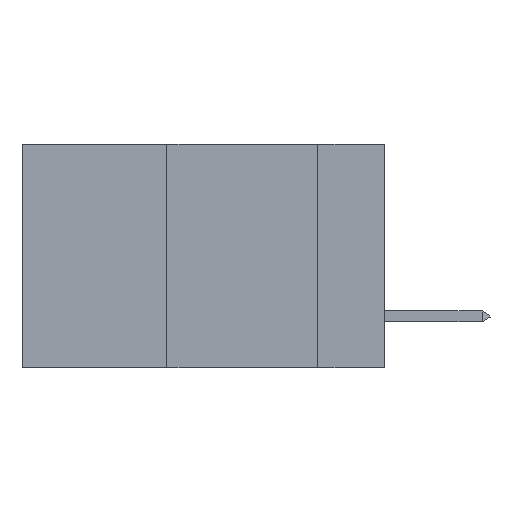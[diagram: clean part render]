
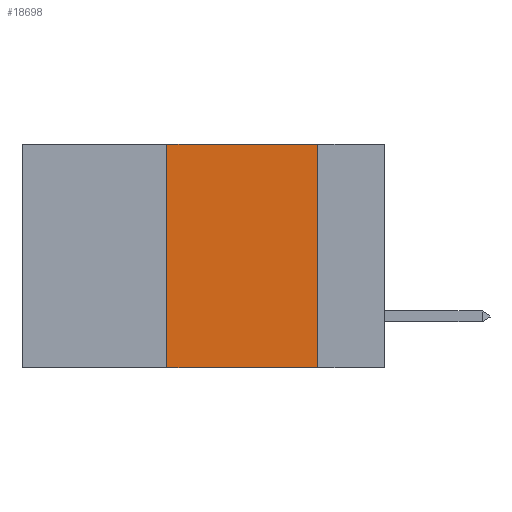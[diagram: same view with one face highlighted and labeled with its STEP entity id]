
A CAD part, left-side view. The second image highlights one B-rep face of the part: STEP entity #18698.
In plain terms, the highlighted planar face has unit normal (-1, 0, 0).
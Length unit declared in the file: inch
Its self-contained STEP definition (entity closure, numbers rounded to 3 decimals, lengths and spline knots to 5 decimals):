
#898 = EDGE_LOOP ( 'NONE', ( #26994, #12466, #18813, #14723 ) ) ;
#1641 = VECTOR ( 'NONE', #14928, 39.37008 ) ;
#2101 = DIRECTION ( 'NONE',  ( 0., -1., 0. ) ) ;
#3492 = CARTESIAN_POINT ( 'NONE',  ( 0., 0.36, 0. ) ) ;
#4423 = PLANE ( 'NONE',  #25157 ) ;
#5091 = VERTEX_POINT ( 'NONE', #13946 ) ;
#5273 = EDGE_CURVE ( 'NONE', #17219, #12558, #10427, .T. ) ;
#7142 = DIRECTION ( 'NONE',  ( 0., 0., -1. ) ) ;
#8526 = VECTOR ( 'NONE', #16353, 39.37008 ) ;
#9247 = CARTESIAN_POINT ( 'NONE',  ( 0., 0.11, -0.37 ) ) ;
#10427 = LINE ( 'NONE', #17237, #1641 ) ;
#12466 = ORIENTED_EDGE ( 'NONE', *, *, #18702, .F. ) ;
#12524 = CARTESIAN_POINT ( 'NONE',  ( 0., 0.6, 0. ) ) ;
#12558 = VERTEX_POINT ( 'NONE', #9247 ) ;
#13273 = CARTESIAN_POINT ( 'NONE',  ( 0., 0.36, 0. ) ) ;
#13766 = VECTOR ( 'NONE', #2101, 39.37008 ) ;
#13946 = CARTESIAN_POINT ( 'NONE',  ( 0., 0.36, -0.37 ) ) ;
#14723 = ORIENTED_EDGE ( 'NONE', *, *, #14860, .T. ) ;
#14860 = EDGE_CURVE ( 'NONE', #5091, #12558, #24760, .T. ) ;
#14928 = DIRECTION ( 'NONE',  ( 0., 0., -1. ) ) ;
#16353 = DIRECTION ( 'NONE',  ( 0., 0., 1. ) ) ;
#17219 = VERTEX_POINT ( 'NONE', #19850 ) ;
#17237 = CARTESIAN_POINT ( 'NONE',  ( 0., 0.11, 0. ) ) ;
#17925 = VECTOR ( 'NONE', #32144, 39.37008 ) ;
#18698 = ADVANCED_FACE ( 'NONE', ( #31250 ), #4423, .F. ) ;
#18702 = EDGE_CURVE ( 'NONE', #21199, #17219, #31284, .T. ) ;
#18813 = ORIENTED_EDGE ( 'NONE', *, *, #19788, .F. ) ;
#19591 = DIRECTION ( 'NONE',  ( 1., 0., 0. ) ) ;
#19788 = EDGE_CURVE ( 'NONE', #5091, #21199, #21705, .T. ) ;
#19850 = CARTESIAN_POINT ( 'NONE',  ( 0., 0.11, 0. ) ) ;
#21199 = VERTEX_POINT ( 'NONE', #13273 ) ;
#21705 = LINE ( 'NONE', #3492, #8526 ) ;
#22310 = CARTESIAN_POINT ( 'NONE',  ( 0., 0.6, 0. ) ) ;
#24760 = LINE ( 'NONE', #32264, #17925 ) ;
#25157 = AXIS2_PLACEMENT_3D ( 'NONE', #12524, #19591, #7142 ) ;
#26994 = ORIENTED_EDGE ( 'NONE', *, *, #5273, .F. ) ;
#31250 = FACE_OUTER_BOUND ( 'NONE', #898, .T. ) ;
#31284 = LINE ( 'NONE', #22310, #13766 ) ;
#32144 = DIRECTION ( 'NONE',  ( 0., -1., 0. ) ) ;
#32264 = CARTESIAN_POINT ( 'NONE',  ( 0., 0.6, -0.37 ) ) ;
